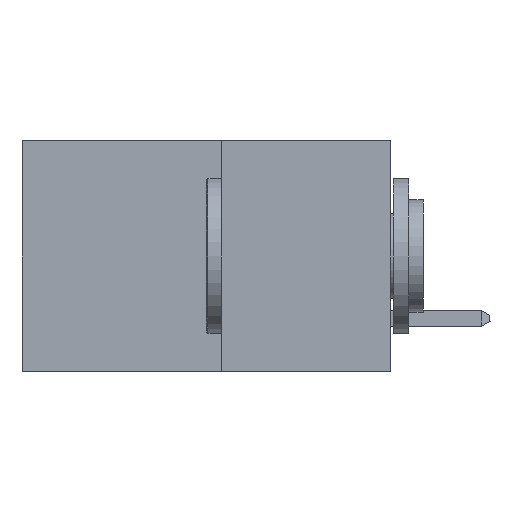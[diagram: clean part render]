
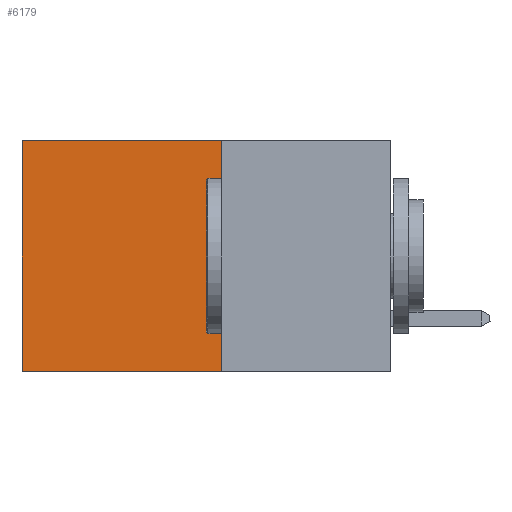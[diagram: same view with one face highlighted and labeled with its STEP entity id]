
A CAD part, left-side view. The second image highlights one B-rep face of the part: STEP entity #6179.
In plain terms, the highlighted planar face has unit normal (-1, 0, 0).
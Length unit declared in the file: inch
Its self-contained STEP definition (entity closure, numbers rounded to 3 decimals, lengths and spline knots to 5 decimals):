
#532 = VECTOR ( 'NONE', #17264, 39.37008 ) ;
#1109 = LINE ( 'NONE', #15369, #532 ) ;
#2208 = CARTESIAN_POINT ( 'NONE',  ( 0.277, 0.27, -0.37 ) ) ;
#2239 = LINE ( 'NONE', #2208, #6633 ) ;
#3686 = DIRECTION ( 'NONE',  ( 0., 1., 0. ) ) ;
#4951 = EDGE_CURVE ( 'NONE', #5704, #15836, #13485, .T. ) ;
#5508 = VECTOR ( 'NONE', #10724, 39.37008 ) ;
#5615 = DIRECTION ( 'NONE',  ( 0., 0., -1. ) ) ;
#5704 = VERTEX_POINT ( 'NONE', #18901 ) ;
#6179 = ADVANCED_FACE ( 'NONE', ( #10998 ), #7074, .F. ) ;
#6575 = CARTESIAN_POINT ( 'NONE',  ( 0.277, 0.59, -0.37 ) ) ;
#6633 = VECTOR ( 'NONE', #5615, 39.37008 ) ;
#6690 = EDGE_LOOP ( 'NONE', ( #8018, #21984, #21542, #19436 ) ) ;
#7074 = PLANE ( 'NONE',  #19938 ) ;
#8018 = ORIENTED_EDGE ( 'NONE', *, *, #19433, .T. ) ;
#8826 = CARTESIAN_POINT ( 'NONE',  ( 0.277, 0.59, -0.37 ) ) ;
#9910 = LINE ( 'NONE', #8826, #5508 ) ;
#10094 = VERTEX_POINT ( 'NONE', #16435 ) ;
#10253 = EDGE_CURVE ( 'NONE', #10094, #22985, #1109, .T. ) ;
#10724 = DIRECTION ( 'NONE',  ( 0., 0., -1. ) ) ;
#10857 = DIRECTION ( 'NONE',  ( 1., 0., 0. ) ) ;
#10998 = FACE_OUTER_BOUND ( 'NONE', #6690, .T. ) ;
#12950 = CARTESIAN_POINT ( 'NONE',  ( 0.277, 0.59, 0. ) ) ;
#13485 = LINE ( 'NONE', #14925, #23469 ) ;
#14925 = CARTESIAN_POINT ( 'NONE',  ( 0.277, 0.27, 0. ) ) ;
#15369 = CARTESIAN_POINT ( 'NONE',  ( 0.277, 0.27, -0.37 ) ) ;
#15836 = VERTEX_POINT ( 'NONE', #12950 ) ;
#16435 = CARTESIAN_POINT ( 'NONE',  ( 0.277, 0.27, -0.37 ) ) ;
#17264 = DIRECTION ( 'NONE',  ( 0., 1., 0. ) ) ;
#18901 = CARTESIAN_POINT ( 'NONE',  ( 0.277, 0.27, 0. ) ) ;
#19433 = EDGE_CURVE ( 'NONE', #15836, #22985, #9910, .T. ) ;
#19436 = ORIENTED_EDGE ( 'NONE', *, *, #4951, .T. ) ;
#19938 = AXIS2_PLACEMENT_3D ( 'NONE', #20222, #10857, #23991 ) ;
#20200 = EDGE_CURVE ( 'NONE', #5704, #10094, #2239, .T. ) ;
#20222 = CARTESIAN_POINT ( 'NONE',  ( 0.277, 0.27, -0.37 ) ) ;
#21542 = ORIENTED_EDGE ( 'NONE', *, *, #20200, .F. ) ;
#21984 = ORIENTED_EDGE ( 'NONE', *, *, #10253, .F. ) ;
#22985 = VERTEX_POINT ( 'NONE', #6575 ) ;
#23469 = VECTOR ( 'NONE', #3686, 39.37008 ) ;
#23991 = DIRECTION ( 'NONE',  ( 0., 0., -1. ) ) ;
